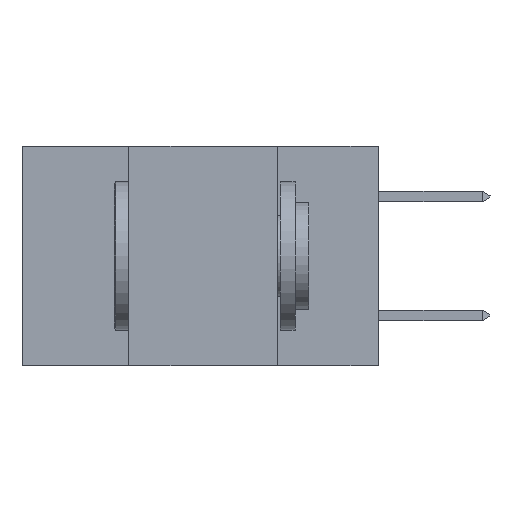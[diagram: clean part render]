
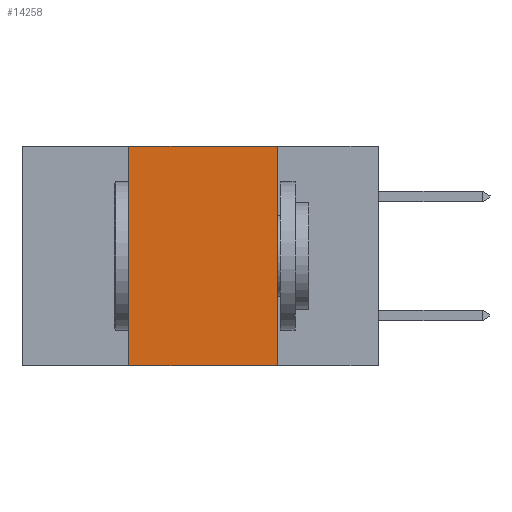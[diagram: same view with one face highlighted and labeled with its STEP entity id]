
A CAD part, left-side view. The second image highlights one B-rep face of the part: STEP entity #14258.
In plain terms, the highlighted planar face has unit normal (-1, 0, 0).
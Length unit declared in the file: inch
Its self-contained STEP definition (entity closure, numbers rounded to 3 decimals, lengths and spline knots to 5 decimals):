
#312 = CARTESIAN_POINT ( 'NONE',  ( 0., 0.42, -0.37 ) ) ;
#580 = CARTESIAN_POINT ( 'NONE',  ( 0., 0.17, -0.37 ) ) ;
#1131 = ORIENTED_EDGE ( 'NONE', *, *, #19137, .F. ) ;
#1624 = DIRECTION ( 'NONE',  ( 0., -1., 0. ) ) ;
#1975 = DIRECTION ( 'NONE',  ( 0., -1., 0. ) ) ;
#2855 = CARTESIAN_POINT ( 'NONE',  ( 0., 0.42, -0.37 ) ) ;
#4173 = AXIS2_PLACEMENT_3D ( 'NONE', #7608, #4439, #10529 ) ;
#4439 = DIRECTION ( 'NONE',  ( 1., 0., 0. ) ) ;
#5152 = EDGE_CURVE ( 'NONE', #16896, #7264, #10660, .T. ) ;
#6006 = VECTOR ( 'NONE', #6608, 39.37008 ) ;
#6087 = VERTEX_POINT ( 'NONE', #15453 ) ;
#6608 = DIRECTION ( 'NONE',  ( 0., 0., -1. ) ) ;
#7264 = VERTEX_POINT ( 'NONE', #18525 ) ;
#7608 = CARTESIAN_POINT ( 'NONE',  ( 0., 0.6, 0. ) ) ;
#8033 = EDGE_LOOP ( 'NONE', ( #11087, #1131, #17562, #18099 ) ) ;
#10529 = DIRECTION ( 'NONE',  ( 0., 0., -1. ) ) ;
#10619 = FACE_OUTER_BOUND ( 'NONE', #8033, .T. ) ;
#10660 = LINE ( 'NONE', #15087, #12359 ) ;
#11087 = ORIENTED_EDGE ( 'NONE', *, *, #19166, .F. ) ;
#11430 = LINE ( 'NONE', #580, #6006 ) ;
#11523 = VERTEX_POINT ( 'NONE', #15130 ) ;
#12359 = VECTOR ( 'NONE', #1624, 39.37008 ) ;
#13236 = DIRECTION ( 'NONE',  ( 0., 0., 1. ) ) ;
#14258 = ADVANCED_FACE ( 'NONE', ( #10619 ), #18161, .F. ) ;
#14643 = VECTOR ( 'NONE', #13236, 39.37008 ) ;
#15087 = CARTESIAN_POINT ( 'NONE',  ( 0., 0.6, -0.37 ) ) ;
#15130 = CARTESIAN_POINT ( 'NONE',  ( 0., 0.17, 0. ) ) ;
#15265 = VECTOR ( 'NONE', #1975, 39.37008 ) ;
#15453 = CARTESIAN_POINT ( 'NONE',  ( 0., 0.42, 0. ) ) ;
#16543 = LINE ( 'NONE', #2855, #14643 ) ;
#16896 = VERTEX_POINT ( 'NONE', #312 ) ;
#17562 = ORIENTED_EDGE ( 'NONE', *, *, #19282, .F. ) ;
#18099 = ORIENTED_EDGE ( 'NONE', *, *, #5152, .T. ) ;
#18161 = PLANE ( 'NONE',  #4173 ) ;
#18525 = CARTESIAN_POINT ( 'NONE',  ( 0., 0.17, -0.37 ) ) ;
#18758 = LINE ( 'NONE', #19047, #15265 ) ;
#19047 = CARTESIAN_POINT ( 'NONE',  ( 0., 0.6, 0. ) ) ;
#19137 = EDGE_CURVE ( 'NONE', #6087, #11523, #18758, .T. ) ;
#19166 = EDGE_CURVE ( 'NONE', #11523, #7264, #11430, .T. ) ;
#19282 = EDGE_CURVE ( 'NONE', #16896, #6087, #16543, .T. ) ;
